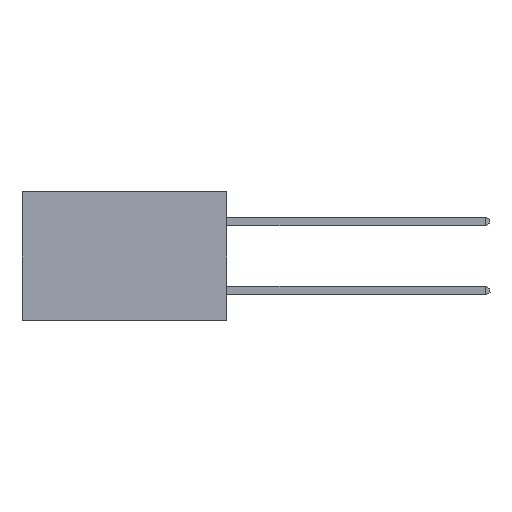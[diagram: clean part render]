
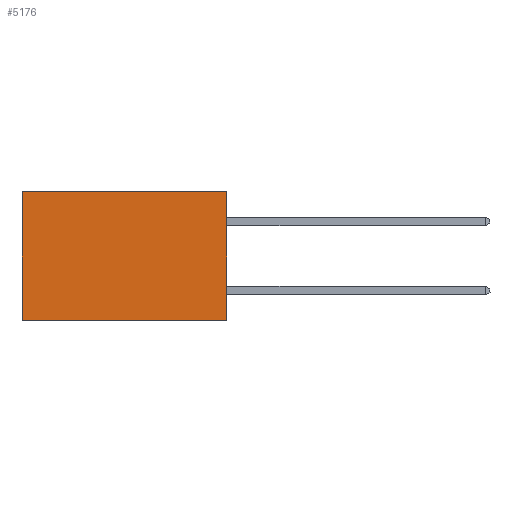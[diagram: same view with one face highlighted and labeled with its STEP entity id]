
A CAD part, left-side view. The second image highlights one B-rep face of the part: STEP entity #5176.
In plain terms, the highlighted planar face has unit normal (-1, 0, 0).
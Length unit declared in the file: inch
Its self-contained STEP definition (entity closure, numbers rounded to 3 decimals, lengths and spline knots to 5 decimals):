
#312 = ORIENTED_EDGE ( 'NONE', *, *, #19246, .T. ) ;
#543 = LINE ( 'NONE', #2471, #10674 ) ;
#748 = VERTEX_POINT ( 'NONE', #20289 ) ;
#1003 = EDGE_LOOP ( 'NONE', ( #18693, #19948, #25164, #312 ) ) ;
#1921 = VERTEX_POINT ( 'NONE', #6106 ) ;
#2349 = AXIS2_PLACEMENT_3D ( 'NONE', #13203, #13139, #13049 ) ;
#2471 = CARTESIAN_POINT ( 'NONE',  ( 0.277, 0., -0.37 ) ) ;
#3009 = VECTOR ( 'NONE', #4865, 39.37008 ) ;
#4865 = DIRECTION ( 'NONE',  ( 0., 1., 0. ) ) ;
#5176 = ADVANCED_FACE ( 'NONE', ( #12328 ), #13288, .F. ) ;
#6106 = CARTESIAN_POINT ( 'NONE',  ( 0.277, 0.59, 0. ) ) ;
#9913 = CARTESIAN_POINT ( 'NONE',  ( 0.277, 0.59, -0.37 ) ) ;
#10674 = VECTOR ( 'NONE', #17218, 39.37008 ) ;
#11221 = CARTESIAN_POINT ( 'NONE',  ( 0.277, 0., -0.37 ) ) ;
#11244 = LINE ( 'NONE', #22549, #16052 ) ;
#12328 = FACE_OUTER_BOUND ( 'NONE', #1003, .T. ) ;
#12359 = DIRECTION ( 'NONE',  ( 0., 0., -1. ) ) ;
#12406 = DIRECTION ( 'NONE',  ( 0., 1., 0. ) ) ;
#12951 = EDGE_CURVE ( 'NONE', #1921, #24746, #15017, .T. ) ;
#13049 = DIRECTION ( 'NONE',  ( 0., 0., -1. ) ) ;
#13139 = DIRECTION ( 'NONE',  ( 1., 0., 0. ) ) ;
#13203 = CARTESIAN_POINT ( 'NONE',  ( 0.277, 0., -0.37 ) ) ;
#13288 = PLANE ( 'NONE',  #2349 ) ;
#13739 = VECTOR ( 'NONE', #12359, 39.37008 ) ;
#14314 = LINE ( 'NONE', #19432, #3009 ) ;
#15017 = LINE ( 'NONE', #26468, #13739 ) ;
#15994 = VERTEX_POINT ( 'NONE', #11221 ) ;
#16052 = VECTOR ( 'NONE', #12406, 39.37008 ) ;
#17218 = DIRECTION ( 'NONE',  ( 0., 0., -1. ) ) ;
#18693 = ORIENTED_EDGE ( 'NONE', *, *, #12951, .T. ) ;
#19246 = EDGE_CURVE ( 'NONE', #748, #1921, #14314, .T. ) ;
#19432 = CARTESIAN_POINT ( 'NONE',  ( 0.277, 0., 0. ) ) ;
#19948 = ORIENTED_EDGE ( 'NONE', *, *, #26579, .F. ) ;
#20289 = CARTESIAN_POINT ( 'NONE',  ( 0.277, 0., 0. ) ) ;
#22458 = EDGE_CURVE ( 'NONE', #748, #15994, #543, .T. ) ;
#22549 = CARTESIAN_POINT ( 'NONE',  ( 0.277, 0., -0.37 ) ) ;
#24746 = VERTEX_POINT ( 'NONE', #9913 ) ;
#25164 = ORIENTED_EDGE ( 'NONE', *, *, #22458, .F. ) ;
#26468 = CARTESIAN_POINT ( 'NONE',  ( 0.277, 0.59, -0.37 ) ) ;
#26579 = EDGE_CURVE ( 'NONE', #15994, #24746, #11244, .T. ) ;
